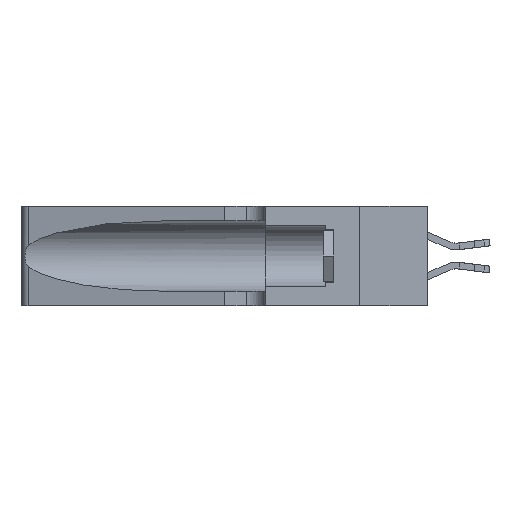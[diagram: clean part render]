
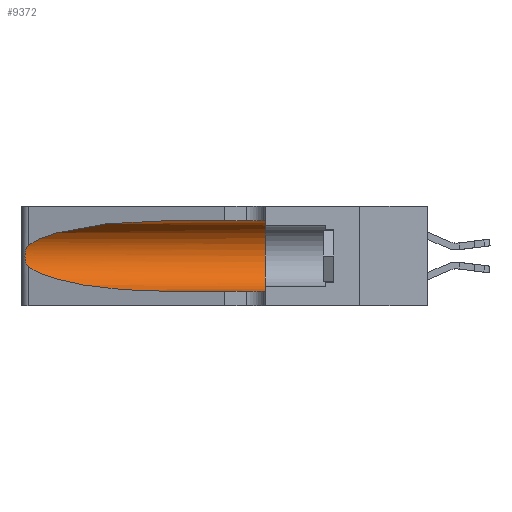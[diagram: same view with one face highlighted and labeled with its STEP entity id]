
A CAD part, left-side view. The second image highlights one B-rep face of the part: STEP entity #9372.
In plain terms, the highlighted cylindrical face has radius 3.308 mm (diameter 6.617 mm), a partial arc.
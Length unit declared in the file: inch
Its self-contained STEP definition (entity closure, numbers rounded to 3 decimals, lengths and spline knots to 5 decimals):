
#28 = EDGE_CURVE ( 'NONE', #32444, #24764, #34292, .T. ) ;
#218 = CYLINDRICAL_SURFACE ( 'NONE', #25523, 0.13025 ) ;
#426 = CARTESIAN_POINT ( 'NONE',  ( 0.25639, 1.23186, 0.15144 ) ) ;
#531 = ORIENTED_EDGE ( 'NONE', *, *, #15370, .T. ) ;
#1299 =( BOUNDED_CURVE ( )  B_SPLINE_CURVE ( 3, ( #10764, #15989, #2112, #30005 ),
 .UNSPECIFIED., .F., .F. ) 
 B_SPLINE_CURVE_WITH_KNOTS ( ( 4, 4 ),
 ( 3.44316, 4.71239 ),
 .UNSPECIFIED. ) 
 CURVE ( )  GEOMETRIC_REPRESENTATION_ITEM ( )  RATIONAL_B_SPLINE_CURVE ( ( 1., 0.87, 0.87, 1. ) ) 
 REPRESENTATION_ITEM ( '' )  );
#1354 = CARTESIAN_POINT ( 'NONE',  ( 0.2373, 1.15595, 0.28018 ) ) ;
#1644 = VERTEX_POINT ( 'NONE', #33457 ) ;
#2112 = CARTESIAN_POINT ( 'NONE',  ( 0.18966, 0.96281, 0.05475 ) ) ;
#3424 = CARTESIAN_POINT ( 'NONE',  ( 0.25487, 1.22718, 0.14631 ) ) ;
#3440 = DIRECTION ( 'NONE',  ( 0., 0., -1. ) ) ;
#3778 = VERTEX_POINT ( 'NONE', #13108 ) ;
#3959 = DIRECTION ( 'NONE',  ( 0., 1., 0. ) ) ;
#6051 = ORIENTED_EDGE ( 'NONE', *, *, #28, .F. ) ;
#6177 = CARTESIAN_POINT ( 'NONE',  ( 0.25639, 1.23184, 0.21858 ) ) ;
#6315 = DIRECTION ( 'NONE',  ( 0., -1., 0. ) ) ;
#6524 = CARTESIAN_POINT ( 'NONE',  ( 0.1305, 0.72297, 0.05475 ) ) ;
#8035 =( BOUNDED_CURVE ( )  B_SPLINE_CURVE ( 3, ( #15537, #31968, #1354, #21075 ),
 .UNSPECIFIED., .F., .T. ) 
 B_SPLINE_CURVE_WITH_KNOTS ( ( 4, 4 ),
 ( 1.5708, 2.84003 ),
 .UNSPECIFIED. ) 
 CURVE ( )  GEOMETRIC_REPRESENTATION_ITEM ( )  RATIONAL_B_SPLINE_CURVE ( ( 1., 0.87, 0.87, 1. ) ) 
 REPRESENTATION_ITEM ( '' )  );
#8842 = FACE_OUTER_BOUND ( 'NONE', #25024, .T. ) ;
#9043 = CARTESIAN_POINT ( 'NONE',  ( 0.25854, 1.2359, 0.20912 ) ) ;
#9151 = ORIENTED_EDGE ( 'NONE', *, *, #31207, .T. ) ;
#9372 = ADVANCED_FACE ( 'NONE', ( #8842 ), #218, .F. ) ;
#10760 = VECTOR ( 'NONE', #32994, 39.37008 ) ;
#10764 = CARTESIAN_POINT ( 'NONE',  ( 0.25487, 1.22718, 0.14631 ) ) ;
#10928 = ORIENTED_EDGE ( 'NONE', *, *, #15833, .T. ) ;
#10989 = CARTESIAN_POINT ( 'NONE',  ( 0.1305, 1.61858, 0.31525 ) ) ;
#11760 = CARTESIAN_POINT ( 'NONE',  ( 0.25555, 1.22994, 0.2215 ) ) ;
#11802 = ORIENTED_EDGE ( 'NONE', *, *, #27234, .T. ) ;
#11881 = CARTESIAN_POINT ( 'NONE',  ( 0.26075, 1.23896, 0.19203 ) ) ;
#13108 = CARTESIAN_POINT ( 'NONE',  ( 0.25487, 1.22718, 0.22369 ) ) ;
#13960 = CARTESIAN_POINT ( 'NONE',  ( 0.1305, 1.61858, 0.05475 ) ) ;
#14393 = LINE ( 'NONE', #13960, #28966 ) ;
#14562 = CARTESIAN_POINT ( 'NONE',  ( 0.25487, 1.22718, 0.22369 ) ) ;
#14677 = CARTESIAN_POINT ( 'NONE',  ( 0.26017, 1.23833, 0.17102 ) ) ;
#15298 = ORIENTED_EDGE ( 'NONE', *, *, #21963, .F. ) ;
#15370 = EDGE_CURVE ( 'NONE', #1644, #3778, #8035, .T. ) ;
#15537 = CARTESIAN_POINT ( 'NONE',  ( 0.1305, 0.72297, 0.31525 ) ) ;
#15833 = EDGE_CURVE ( 'NONE', #20866, #30736, #1299, .T. ) ;
#15989 = CARTESIAN_POINT ( 'NONE',  ( 0.2373, 1.15595, 0.08982 ) ) ;
#17470 = CARTESIAN_POINT ( 'NONE',  ( 0.25789, 1.23486, 0.15765 ) ) ;
#20230 = CARTESIAN_POINT ( 'NONE',  ( 0.25555, 1.22993, 0.14849 ) ) ;
#20866 = VERTEX_POINT ( 'NONE', #33635 ) ;
#21075 = CARTESIAN_POINT ( 'NONE',  ( 0.25487, 1.22718, 0.22369 ) ) ;
#21963 = EDGE_CURVE ( 'NONE', #1644, #32444, #25401, .T. ) ;
#22775 = CARTESIAN_POINT ( 'NONE',  ( 0.1305, 0.35, 0.31525 ) ) ;
#22978 = CARTESIAN_POINT ( 'NONE',  ( 0.1305, 1.61858, 0.185 ) ) ;
#24764 = VERTEX_POINT ( 'NONE', #30915 ) ;
#24908 = AXIS2_PLACEMENT_3D ( 'NONE', #29767, #3959, #28581 ) ;
#25024 = EDGE_LOOP ( 'NONE', ( #531, #9151, #10928, #11802, #6051, #15298 ) ) ;
#25401 = LINE ( 'NONE', #10989, #10760 ) ;
#25523 = AXIS2_PLACEMENT_3D ( 'NONE', #22978, #6315, #3440 ) ;
#25589 = CARTESIAN_POINT ( 'NONE',  ( 0.25787, 1.23484, 0.2124 ) ) ;
#27234 = EDGE_CURVE ( 'NONE', #30736, #24764, #14393, .T. ) ;
#28326 = CARTESIAN_POINT ( 'NONE',  ( 0.26018, 1.23835, 0.19895 ) ) ;
#28385 = B_SPLINE_CURVE_WITH_KNOTS ( 'NONE', 3,
 ( #14562, #11760, #6177, #25589, #9043, #28326, #11881, #31114, #14677, #33865, #17470, #426, #20230, #3424 ),
 .UNSPECIFIED., .F., .F.,
 ( 4, 2, 2, 2, 2, 2, 4 ),
 ( 0., 0.00027, 0.00053, 0.00107, 0.0016, 0.00187, 0.00214 ),
 .UNSPECIFIED. ) ;
#28581 = DIRECTION ( 'NONE',  ( 0., 0., 1. ) ) ;
#28966 = VECTOR ( 'NONE', #35772, 39.37008 ) ;
#29767 = CARTESIAN_POINT ( 'NONE',  ( 0.1305, 0.35, 0.185 ) ) ;
#30005 = CARTESIAN_POINT ( 'NONE',  ( 0.1305, 0.72297, 0.05475 ) ) ;
#30736 = VERTEX_POINT ( 'NONE', #6524 ) ;
#30915 = CARTESIAN_POINT ( 'NONE',  ( 0.1305, 0.35, 0.05475 ) ) ;
#31114 = CARTESIAN_POINT ( 'NONE',  ( 0.26075, 1.23896, 0.178 ) ) ;
#31207 = EDGE_CURVE ( 'NONE', #3778, #20866, #28385, .T. ) ;
#31968 = CARTESIAN_POINT ( 'NONE',  ( 0.18966, 0.96281, 0.31525 ) ) ;
#32444 = VERTEX_POINT ( 'NONE', #22775 ) ;
#32994 = DIRECTION ( 'NONE',  ( 0., -1., 0. ) ) ;
#33457 = CARTESIAN_POINT ( 'NONE',  ( 0.1305, 0.72297, 0.31525 ) ) ;
#33635 = CARTESIAN_POINT ( 'NONE',  ( 0.25487, 1.22718, 0.14631 ) ) ;
#33865 = CARTESIAN_POINT ( 'NONE',  ( 0.25856, 1.23593, 0.16098 ) ) ;
#34292 = CIRCLE ( 'NONE', #24908, 0.13025 ) ;
#35772 = DIRECTION ( 'NONE',  ( 0., -1., 0. ) ) ;
